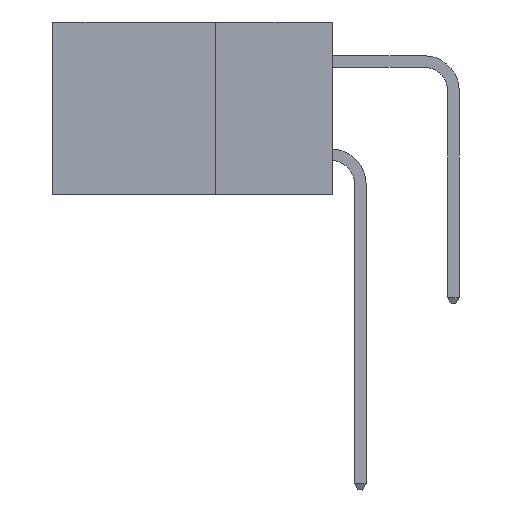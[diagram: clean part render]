
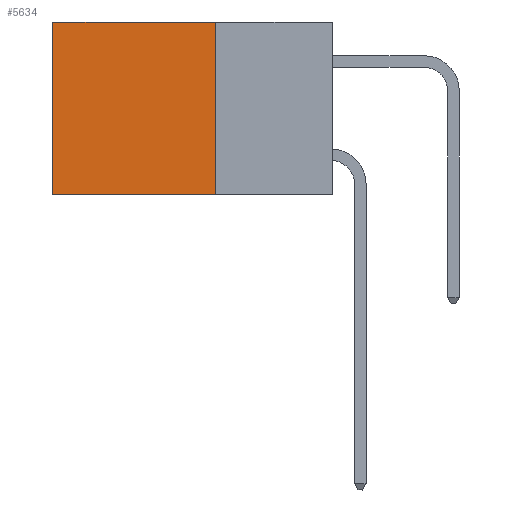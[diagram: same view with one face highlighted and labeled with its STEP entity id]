
A CAD part, left-side view. The second image highlights one B-rep face of the part: STEP entity #5634.
In plain terms, the highlighted planar face has unit normal (-1, 0, 0).
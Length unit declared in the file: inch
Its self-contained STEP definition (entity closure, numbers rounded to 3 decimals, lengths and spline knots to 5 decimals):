
#83 = DIRECTION ( 'NONE',  ( 0., 1., 0. ) ) ;
#104 = LINE ( 'NONE', #1746, #5378 ) ;
#652 = ORIENTED_EDGE ( 'NONE', *, *, #1423, .T. ) ;
#1168 = PLANE ( 'NONE',  #6877 ) ;
#1423 = EDGE_CURVE ( 'NONE', #2507, #11470, #2984, .T. ) ;
#1746 = CARTESIAN_POINT ( 'NONE',  ( 0.298, 0.25, 0. ) ) ;
#2005 = DIRECTION ( 'NONE',  ( 0., 0., -1. ) ) ;
#2083 = VECTOR ( 'NONE', #16592, 39.37008 ) ;
#2332 = CARTESIAN_POINT ( 'NONE',  ( 0.298, 0.25, -0.37 ) ) ;
#2507 = VERTEX_POINT ( 'NONE', #18214 ) ;
#2830 = CARTESIAN_POINT ( 'NONE',  ( 0.298, 0.25, 0. ) ) ;
#2984 = LINE ( 'NONE', #13686, #2083 ) ;
#4190 = ORIENTED_EDGE ( 'NONE', *, *, #11685, .F. ) ;
#4302 = DIRECTION ( 'NONE',  ( 1., 0., 0. ) ) ;
#4973 = VECTOR ( 'NONE', #15394, 39.37008 ) ;
#5378 = VECTOR ( 'NONE', #83, 39.37008 ) ;
#5634 = ADVANCED_FACE ( 'NONE', ( #11018 ), #1168, .F. ) ;
#6877 = AXIS2_PLACEMENT_3D ( 'NONE', #2830, #4302, #7128 ) ;
#7128 = DIRECTION ( 'NONE',  ( 0., 0., -1. ) ) ;
#8384 = ORIENTED_EDGE ( 'NONE', *, *, #11706, .F. ) ;
#8762 = CARTESIAN_POINT ( 'NONE',  ( 0.298, 0.25, -0.37 ) ) ;
#9448 = VERTEX_POINT ( 'NONE', #2332 ) ;
#10257 = VECTOR ( 'NONE', #2005, 39.37008 ) ;
#10730 = CARTESIAN_POINT ( 'NONE',  ( 0.298, 0.25, 0. ) ) ;
#11018 = FACE_OUTER_BOUND ( 'NONE', #14225, .T. ) ;
#11389 = LINE ( 'NONE', #14441, #10257 ) ;
#11470 = VERTEX_POINT ( 'NONE', #16902 ) ;
#11685 = EDGE_CURVE ( 'NONE', #9448, #11470, #18862, .T. ) ;
#11706 = EDGE_CURVE ( 'NONE', #14937, #9448, #11389, .T. ) ;
#13686 = CARTESIAN_POINT ( 'NONE',  ( 0.298, 0.6, 0. ) ) ;
#14225 = EDGE_LOOP ( 'NONE', ( #652, #4190, #8384, #16964 ) ) ;
#14441 = CARTESIAN_POINT ( 'NONE',  ( 0.298, 0.25, 0. ) ) ;
#14937 = VERTEX_POINT ( 'NONE', #10730 ) ;
#15394 = DIRECTION ( 'NONE',  ( 0., 1., 0. ) ) ;
#16592 = DIRECTION ( 'NONE',  ( 0., 0., -1. ) ) ;
#16902 = CARTESIAN_POINT ( 'NONE',  ( 0.298, 0.6, -0.37 ) ) ;
#16964 = ORIENTED_EDGE ( 'NONE', *, *, #17267, .T. ) ;
#17267 = EDGE_CURVE ( 'NONE', #14937, #2507, #104, .T. ) ;
#18214 = CARTESIAN_POINT ( 'NONE',  ( 0.298, 0.6, 0. ) ) ;
#18862 = LINE ( 'NONE', #8762, #4973 ) ;
